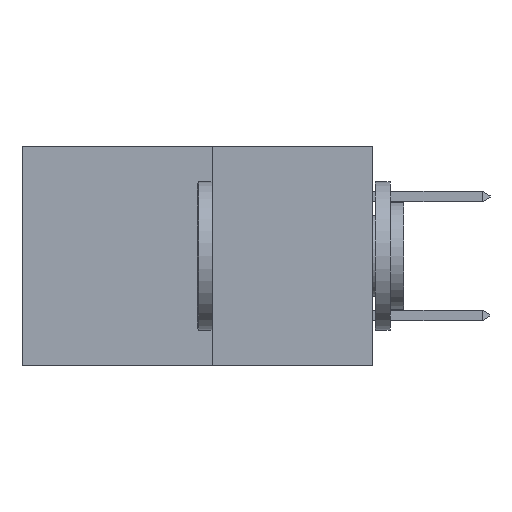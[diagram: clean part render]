
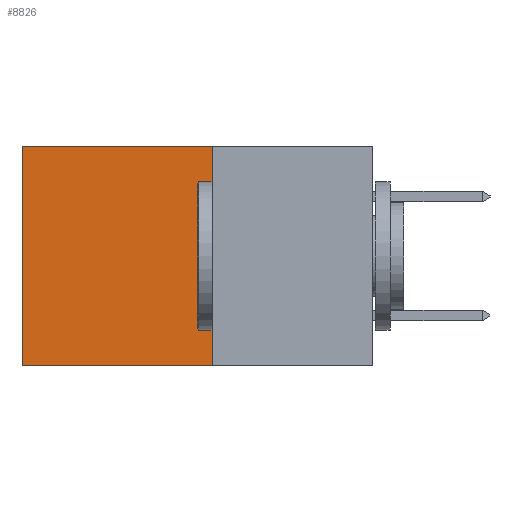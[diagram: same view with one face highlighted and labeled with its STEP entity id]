
A CAD part, left-side view. The second image highlights one B-rep face of the part: STEP entity #8826.
In plain terms, the highlighted planar face has unit normal (-1, 0, 0).
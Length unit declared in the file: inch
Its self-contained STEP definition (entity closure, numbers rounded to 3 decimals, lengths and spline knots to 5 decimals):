
#20 = DIRECTION ( 'NONE',  ( 0., 0., -1. ) ) ;
#202 = CARTESIAN_POINT ( 'NONE',  ( 0.277, 0.59, -0.37 ) ) ;
#282 = CARTESIAN_POINT ( 'NONE',  ( 0.277, 0.59, 0. ) ) ;
#333 = VECTOR ( 'NONE', #2543, 39.37008 ) ;
#617 = CARTESIAN_POINT ( 'NONE',  ( 0.277, 0.27, 0. ) ) ;
#1203 = CARTESIAN_POINT ( 'NONE',  ( 0.277, 0.27, -0.37 ) ) ;
#1338 = FACE_OUTER_BOUND ( 'NONE', #15391, .T. ) ;
#1602 = LINE ( 'NONE', #202, #4692 ) ;
#1909 = PLANE ( 'NONE',  #15318 ) ;
#2315 = VERTEX_POINT ( 'NONE', #12101 ) ;
#2543 = DIRECTION ( 'NONE',  ( 0., 0., -1. ) ) ;
#3637 = VERTEX_POINT ( 'NONE', #282 ) ;
#4241 = ORIENTED_EDGE ( 'NONE', *, *, #5208, .T. ) ;
#4320 = ORIENTED_EDGE ( 'NONE', *, *, #14557, .F. ) ;
#4570 = ORIENTED_EDGE ( 'NONE', *, *, #10691, .F. ) ;
#4692 = VECTOR ( 'NONE', #20, 39.37008 ) ;
#4941 = ORIENTED_EDGE ( 'NONE', *, *, #16148, .T. ) ;
#5208 = EDGE_CURVE ( 'NONE', #3637, #2315, #1602, .T. ) ;
#5872 = CARTESIAN_POINT ( 'NONE',  ( 0.277, 0.27, -0.37 ) ) ;
#6546 = VERTEX_POINT ( 'NONE', #15580 ) ;
#6712 = VERTEX_POINT ( 'NONE', #10979 ) ;
#7169 = DIRECTION ( 'NONE',  ( 0., 0., -1. ) ) ;
#7237 = LINE ( 'NONE', #1203, #333 ) ;
#7524 = LINE ( 'NONE', #11448, #14114 ) ;
#8826 = ADVANCED_FACE ( 'NONE', ( #1338 ), #1909, .F. ) ;
#9626 = DIRECTION ( 'NONE',  ( 0., 1., 0. ) ) ;
#10237 = DIRECTION ( 'NONE',  ( 0., 1., 0. ) ) ;
#10569 = LINE ( 'NONE', #617, #16365 ) ;
#10691 = EDGE_CURVE ( 'NONE', #6546, #6712, #7237, .T. ) ;
#10979 = CARTESIAN_POINT ( 'NONE',  ( 0.277, 0.27, -0.37 ) ) ;
#11448 = CARTESIAN_POINT ( 'NONE',  ( 0.277, 0.27, -0.37 ) ) ;
#12101 = CARTESIAN_POINT ( 'NONE',  ( 0.277, 0.59, -0.37 ) ) ;
#14114 = VECTOR ( 'NONE', #10237, 39.37008 ) ;
#14557 = EDGE_CURVE ( 'NONE', #6712, #2315, #7524, .T. ) ;
#14599 = DIRECTION ( 'NONE',  ( 1., 0., 0. ) ) ;
#15318 = AXIS2_PLACEMENT_3D ( 'NONE', #5872, #14599, #7169 ) ;
#15391 = EDGE_LOOP ( 'NONE', ( #4241, #4320, #4570, #4941 ) ) ;
#15580 = CARTESIAN_POINT ( 'NONE',  ( 0.277, 0.27, 0. ) ) ;
#16148 = EDGE_CURVE ( 'NONE', #6546, #3637, #10569, .T. ) ;
#16365 = VECTOR ( 'NONE', #9626, 39.37008 ) ;
